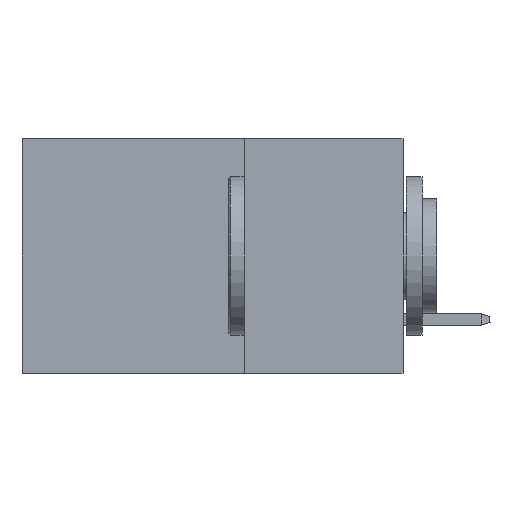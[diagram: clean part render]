
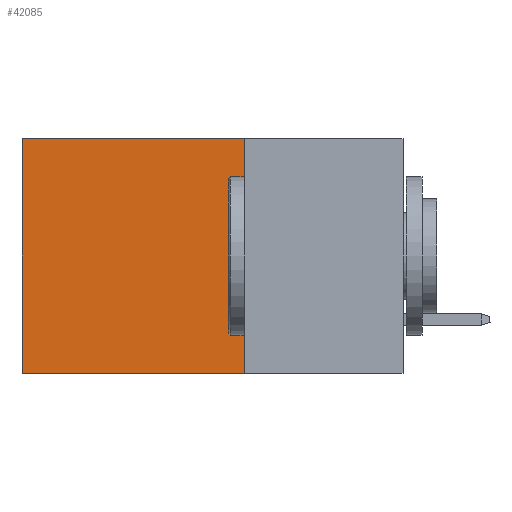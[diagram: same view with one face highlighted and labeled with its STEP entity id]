
A CAD part, left-side view. The second image highlights one B-rep face of the part: STEP entity #42085.
In plain terms, the highlighted planar face has unit normal (-1, 0, 0).
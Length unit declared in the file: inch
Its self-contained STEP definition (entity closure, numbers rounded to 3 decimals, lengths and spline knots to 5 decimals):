
#569 = AXIS2_PLACEMENT_3D ( 'NONE', #23366, #36644, #33220 ) ;
#630 = LINE ( 'NONE', #6177, #41173 ) ;
#2664 = ORIENTED_EDGE ( 'NONE', *, *, #34958, .T. ) ;
#4052 = LINE ( 'NONE', #23903, #29314 ) ;
#6177 = CARTESIAN_POINT ( 'NONE',  ( 0.2875, 0.25, -0.37 ) ) ;
#6331 = VERTEX_POINT ( 'NONE', #31122 ) ;
#7535 = VERTEX_POINT ( 'NONE', #8472 ) ;
#8472 = CARTESIAN_POINT ( 'NONE',  ( 0.2875, 0.25, -0.37 ) ) ;
#9537 = EDGE_CURVE ( 'NONE', #22660, #29316, #42186, .T. ) ;
#10321 = DIRECTION ( 'NONE',  ( 0., 0., -1. ) ) ;
#10440 = CARTESIAN_POINT ( 'NONE',  ( 0.2875, 0.6, 0. ) ) ;
#12314 = LINE ( 'NONE', #35195, #22527 ) ;
#12635 = EDGE_LOOP ( 'NONE', ( #23396, #24677, #22246, #2664 ) ) ;
#15327 = DIRECTION ( 'NONE',  ( 0., 0., -1. ) ) ;
#19204 = DIRECTION ( 'NONE',  ( 0., 1., 0. ) ) ;
#22246 = ORIENTED_EDGE ( 'NONE', *, *, #37400, .F. ) ;
#22527 = VECTOR ( 'NONE', #15327, 39.37008 ) ;
#22660 = VERTEX_POINT ( 'NONE', #10440 ) ;
#23366 = CARTESIAN_POINT ( 'NONE',  ( 0.2875, 0.25, 0. ) ) ;
#23396 = ORIENTED_EDGE ( 'NONE', *, *, #9537, .T. ) ;
#23903 = CARTESIAN_POINT ( 'NONE',  ( 0.2875, 0.25, 0. ) ) ;
#24677 = ORIENTED_EDGE ( 'NONE', *, *, #40236, .F. ) ;
#26239 = CARTESIAN_POINT ( 'NONE',  ( 0.2875, 0.6, -0.37 ) ) ;
#26794 = FACE_OUTER_BOUND ( 'NONE', #12635, .T. ) ;
#29314 = VECTOR ( 'NONE', #33551, 39.37008 ) ;
#29316 = VERTEX_POINT ( 'NONE', #26239 ) ;
#31122 = CARTESIAN_POINT ( 'NONE',  ( 0.2875, 0.25, 0. ) ) ;
#33220 = DIRECTION ( 'NONE',  ( 0., 0., -1. ) ) ;
#33551 = DIRECTION ( 'NONE',  ( 0., 1., 0. ) ) ;
#34958 = EDGE_CURVE ( 'NONE', #6331, #22660, #4052, .T. ) ;
#35195 = CARTESIAN_POINT ( 'NONE',  ( 0.2875, 0.25, 0. ) ) ;
#36644 = DIRECTION ( 'NONE',  ( 1., 0., 0. ) ) ;
#37400 = EDGE_CURVE ( 'NONE', #6331, #7535, #12314, .T. ) ;
#38995 = CARTESIAN_POINT ( 'NONE',  ( 0.2875, 0.6, 0. ) ) ;
#39642 = VECTOR ( 'NONE', #10321, 39.37008 ) ;
#40052 = PLANE ( 'NONE',  #569 ) ;
#40236 = EDGE_CURVE ( 'NONE', #7535, #29316, #630, .T. ) ;
#41173 = VECTOR ( 'NONE', #19204, 39.37008 ) ;
#42085 = ADVANCED_FACE ( 'NONE', ( #26794 ), #40052, .F. ) ;
#42186 = LINE ( 'NONE', #38995, #39642 ) ;
